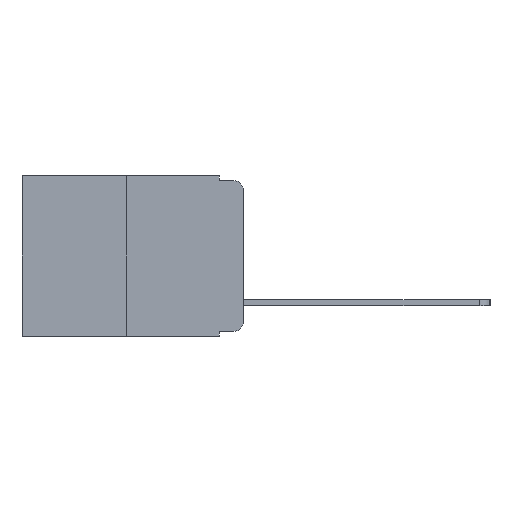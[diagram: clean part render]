
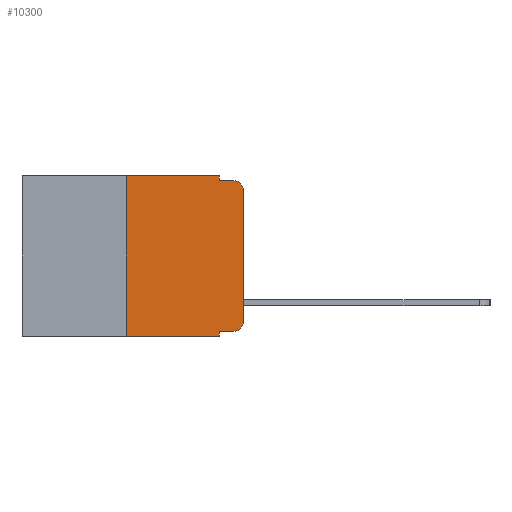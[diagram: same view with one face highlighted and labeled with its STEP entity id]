
A CAD part, left-side view. The second image highlights one B-rep face of the part: STEP entity #10300.
In plain terms, the highlighted planar face has unit normal (-1, 0, 0).
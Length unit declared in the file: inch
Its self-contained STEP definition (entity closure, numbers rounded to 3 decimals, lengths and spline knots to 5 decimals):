
#213 = CARTESIAN_POINT ( 'NONE',  ( 0., 0.473, 0. ) ) ;
#413 = CARTESIAN_POINT ( 'NONE',  ( 0., 0., 0. ) ) ;
#571 = CARTESIAN_POINT ( 'NONE',  ( 0., 0.473, 0. ) ) ;
#604 = DIRECTION ( 'NONE',  ( 0., -1., 0. ) ) ;
#1507 = ORIENTED_EDGE ( 'NONE', *, *, #17029, .T. ) ;
#1835 = VERTEX_POINT ( 'NONE', #6836 ) ;
#2213 = CARTESIAN_POINT ( 'NONE',  ( 0., 0.473, -0.343 ) ) ;
#2249 = LINE ( 'NONE', #2213, #13378 ) ;
#2260 = CARTESIAN_POINT ( 'NONE',  ( 0., 0.02, -0.333 ) ) ;
#2609 = EDGE_CURVE ( 'NONE', #2820, #19192, #2249, .T. ) ;
#2686 = VERTEX_POINT ( 'NONE', #2260 ) ;
#2820 = VERTEX_POINT ( 'NONE', #14489 ) ;
#2999 = CARTESIAN_POINT ( 'NONE',  ( 0., 0.051, -0.01 ) ) ;
#3205 = EDGE_CURVE ( 'NONE', #9464, #8480, #7781, .T. ) ;
#3520 = CARTESIAN_POINT ( 'NONE',  ( 0., 0.051, -0.343 ) ) ;
#3610 = DIRECTION ( 'NONE',  ( 1., 0., 0. ) ) ;
#3621 = ORIENTED_EDGE ( 'NONE', *, *, #13633, .F. ) ;
#4128 = CIRCLE ( 'NONE', #15070, 0.02 ) ;
#4428 = DIRECTION ( 'NONE',  ( 0., 0., 1. ) ) ;
#4519 = FACE_OUTER_BOUND ( 'NONE', #15135, .T. ) ;
#4751 = VECTOR ( 'NONE', #5761, 39.37008 ) ;
#4807 = EDGE_CURVE ( 'NONE', #13721, #8480, #16521, .T. ) ;
#5122 = ORIENTED_EDGE ( 'NONE', *, *, #8221, .T. ) ;
#5761 = DIRECTION ( 'NONE',  ( 0., -1., 0. ) ) ;
#5872 = ORIENTED_EDGE ( 'NONE', *, *, #3205, .T. ) ;
#5937 = DIRECTION ( 'NONE',  ( -1., 0., 0. ) ) ;
#5968 = CARTESIAN_POINT ( 'NONE',  ( 0., 0.25, 0. ) ) ;
#6343 = ORIENTED_EDGE ( 'NONE', *, *, #4807, .F. ) ;
#6836 = CARTESIAN_POINT ( 'NONE',  ( 0., 0.051, -0.333 ) ) ;
#7098 = CARTESIAN_POINT ( 'NONE',  ( 0., 0., -0.313 ) ) ;
#7758 = CARTESIAN_POINT ( 'NONE',  ( 0., 0.051, 0. ) ) ;
#7781 = CIRCLE ( 'NONE', #15098, 0.02 ) ;
#8072 = LINE ( 'NONE', #413, #13842 ) ;
#8221 = EDGE_CURVE ( 'NONE', #2686, #8959, #4128, .T. ) ;
#8349 = CARTESIAN_POINT ( 'NONE',  ( 0., 0.25, 0. ) ) ;
#8368 = ORIENTED_EDGE ( 'NONE', *, *, #2609, .T. ) ;
#8432 = PLANE ( 'NONE',  #16458 ) ;
#8480 = VERTEX_POINT ( 'NONE', #11846 ) ;
#8511 = LINE ( 'NONE', #14986, #4751 ) ;
#8867 = ORIENTED_EDGE ( 'NONE', *, *, #11347, .F. ) ;
#8959 = VERTEX_POINT ( 'NONE', #7098 ) ;
#9227 = VECTOR ( 'NONE', #11797, 39.37008 ) ;
#9464 = VERTEX_POINT ( 'NONE', #13497 ) ;
#9676 = VECTOR ( 'NONE', #4428, 39.37008 ) ;
#10300 = ADVANCED_FACE ( 'NONE', ( #4519 ), #8432, .F. ) ;
#10915 = VERTEX_POINT ( 'NONE', #8349 ) ;
#11153 = EDGE_CURVE ( 'NONE', #1835, #2686, #8511, .T. ) ;
#11347 = EDGE_CURVE ( 'NONE', #1835, #19192, #17208, .T. ) ;
#11536 = ORIENTED_EDGE ( 'NONE', *, *, #15249, .F. ) ;
#11797 = DIRECTION ( 'NONE',  ( 0., -1., 0. ) ) ;
#11846 = CARTESIAN_POINT ( 'NONE',  ( 0., 0.02, -0.01 ) ) ;
#12027 = CARTESIAN_POINT ( 'NONE',  ( 0., 0.051, -0.01 ) ) ;
#12200 = DIRECTION ( 'NONE',  ( -1., 0., 0. ) ) ;
#12396 = CARTESIAN_POINT ( 'NONE',  ( 0., 0.02, -0.03 ) ) ;
#13051 = DIRECTION ( 'NONE',  ( 0., 0., -1. ) ) ;
#13226 = CARTESIAN_POINT ( 'NONE',  ( 0., 0.051, 0. ) ) ;
#13311 = VECTOR ( 'NONE', #16843, 39.37008 ) ;
#13378 = VECTOR ( 'NONE', #604, 39.37008 ) ;
#13497 = CARTESIAN_POINT ( 'NONE',  ( 0., 0., -0.03 ) ) ;
#13633 = EDGE_CURVE ( 'NONE', #2820, #10915, #13704, .T. ) ;
#13704 = LINE ( 'NONE', #5968, #9676 ) ;
#13721 = VERTEX_POINT ( 'NONE', #2999 ) ;
#13842 = VECTOR ( 'NONE', #18988, 39.37008 ) ;
#14489 = CARTESIAN_POINT ( 'NONE',  ( 0., 0.25, -0.343 ) ) ;
#14567 = ORIENTED_EDGE ( 'NONE', *, *, #18858, .F. ) ;
#14986 = CARTESIAN_POINT ( 'NONE',  ( 0., 0.051, -0.333 ) ) ;
#15056 = LINE ( 'NONE', #571, #18036 ) ;
#15070 = AXIS2_PLACEMENT_3D ( 'NONE', #15165, #5937, #16637 ) ;
#15098 = AXIS2_PLACEMENT_3D ( 'NONE', #12396, #12200, #13051 ) ;
#15135 = EDGE_LOOP ( 'NONE', ( #1507, #5872, #6343, #14567, #11536, #3621, #8368, #8867, #16871, #5122 ) ) ;
#15165 = CARTESIAN_POINT ( 'NONE',  ( 0., 0.02, -0.313 ) ) ;
#15249 = EDGE_CURVE ( 'NONE', #10915, #17891, #15056, .T. ) ;
#16065 = VECTOR ( 'NONE', #19548, 39.37008 ) ;
#16458 = AXIS2_PLACEMENT_3D ( 'NONE', #213, #3610, #18887 ) ;
#16521 = LINE ( 'NONE', #12027, #9227 ) ;
#16540 = LINE ( 'NONE', #18148, #16065 ) ;
#16637 = DIRECTION ( 'NONE',  ( 0., 0., -1. ) ) ;
#16843 = DIRECTION ( 'NONE',  ( 0., 0., -1. ) ) ;
#16871 = ORIENTED_EDGE ( 'NONE', *, *, #11153, .T. ) ;
#17029 = EDGE_CURVE ( 'NONE', #8959, #9464, #8072, .T. ) ;
#17208 = LINE ( 'NONE', #7758, #13311 ) ;
#17684 = DIRECTION ( 'NONE',  ( 0., -1., 0. ) ) ;
#17891 = VERTEX_POINT ( 'NONE', #13226 ) ;
#18036 = VECTOR ( 'NONE', #17684, 39.37008 ) ;
#18148 = CARTESIAN_POINT ( 'NONE',  ( 0., 0.051, 0. ) ) ;
#18858 = EDGE_CURVE ( 'NONE', #17891, #13721, #16540, .T. ) ;
#18887 = DIRECTION ( 'NONE',  ( 0., 0., -1. ) ) ;
#18988 = DIRECTION ( 'NONE',  ( 0., 0., 1. ) ) ;
#19192 = VERTEX_POINT ( 'NONE', #3520 ) ;
#19548 = DIRECTION ( 'NONE',  ( 0., 0., -1. ) ) ;
